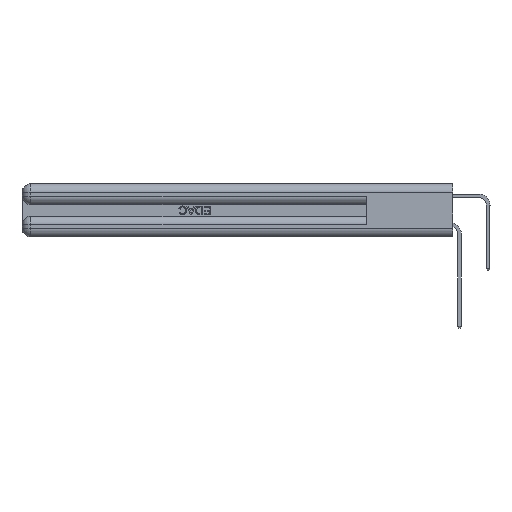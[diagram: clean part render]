
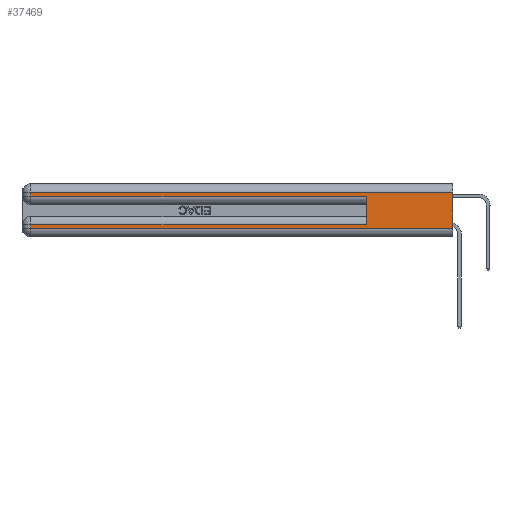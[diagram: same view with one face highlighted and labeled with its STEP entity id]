
A CAD part, left-side view. The second image highlights one B-rep face of the part: STEP entity #37469.
In plain terms, the highlighted planar face has unit normal (-1, 0, 0).
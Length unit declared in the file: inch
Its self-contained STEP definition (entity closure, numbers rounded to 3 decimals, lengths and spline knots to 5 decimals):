
#248 = ORIENTED_EDGE ( 'NONE', *, *, #15402, .T. ) ;
#1178 = ORIENTED_EDGE ( 'NONE', *, *, #9629, .F. ) ;
#1472 = DIRECTION ( 'NONE',  ( 0., 0., -1. ) ) ;
#2189 = EDGE_LOOP ( 'NONE', ( #30689, #19698, #20107, #3870, #1178, #43387, #22085, #248 ) ) ;
#2551 = VERTEX_POINT ( 'NONE', #20019 ) ;
#3870 = ORIENTED_EDGE ( 'NONE', *, *, #19183, .T. ) ;
#5014 = DIRECTION ( 'NONE',  ( 0., -1., 0. ) ) ;
#5498 = VECTOR ( 'NONE', #5014, 39.37008 ) ;
#5734 = CARTESIAN_POINT ( 'NONE',  ( 0., 0., 0.285 ) ) ;
#5761 = CARTESIAN_POINT ( 'NONE',  ( 0., 2.94, 0.31 ) ) ;
#8017 = EDGE_CURVE ( 'NONE', #36345, #47093, #17078, .T. ) ;
#8285 = VECTOR ( 'NONE', #9506, 39.37008 ) ;
#9245 = CARTESIAN_POINT ( 'NONE',  ( 0., 0., 0.37 ) ) ;
#9506 = DIRECTION ( 'NONE',  ( 0., -1., 0. ) ) ;
#9629 = EDGE_CURVE ( 'NONE', #18094, #2551, #47609, .T. ) ;
#10509 = LINE ( 'NONE', #9245, #39495 ) ;
#10948 = VERTEX_POINT ( 'NONE', #39582 ) ;
#11577 = PLANE ( 'NONE',  #39052 ) ;
#11894 = DIRECTION ( 'NONE',  ( 0., 0., -1. ) ) ;
#13617 = EDGE_CURVE ( 'NONE', #10948, #30044, #10509, .T. ) ;
#14584 = DIRECTION ( 'NONE',  ( 0., 0., -1. ) ) ;
#14657 = DIRECTION ( 'NONE',  ( 0., 0., -1. ) ) ;
#15069 = VECTOR ( 'NONE', #44785, 39.37008 ) ;
#15402 = EDGE_CURVE ( 'NONE', #47093, #30044, #16770, .T. ) ;
#16770 = LINE ( 'NONE', #46669, #5498 ) ;
#17068 = CARTESIAN_POINT ( 'NONE',  ( 0., 2.94, 0.085 ) ) ;
#17078 = LINE ( 'NONE', #34968, #21237 ) ;
#17188 = LINE ( 'NONE', #5734, #8285 ) ;
#17857 = CARTESIAN_POINT ( 'NONE',  ( 0., 2.94, 0.06 ) ) ;
#18094 = VERTEX_POINT ( 'NONE', #32365 ) ;
#19183 = EDGE_CURVE ( 'NONE', #25892, #2551, #17188, .T. ) ;
#19698 = ORIENTED_EDGE ( 'NONE', *, *, #41065, .T. ) ;
#20019 = CARTESIAN_POINT ( 'NONE',  ( 0., 0.6, 0.285 ) ) ;
#20107 = ORIENTED_EDGE ( 'NONE', *, *, #40357, .T. ) ;
#21237 = VECTOR ( 'NONE', #14657, 39.37008 ) ;
#21428 = VERTEX_POINT ( 'NONE', #5761 ) ;
#22085 = ORIENTED_EDGE ( 'NONE', *, *, #8017, .T. ) ;
#22688 = CARTESIAN_POINT ( 'NONE',  ( 0., 2.94, 0.285 ) ) ;
#22789 = LINE ( 'NONE', #37031, #15069 ) ;
#23026 = CARTESIAN_POINT ( 'NONE',  ( 0., 0., 0.37 ) ) ;
#23194 = DIRECTION ( 'NONE',  ( 1., 0., 0. ) ) ;
#24087 = DIRECTION ( 'NONE',  ( 0., 1., 0. ) ) ;
#25892 = VERTEX_POINT ( 'NONE', #22688 ) ;
#27527 = LINE ( 'NONE', #45000, #47105 ) ;
#30044 = VERTEX_POINT ( 'NONE', #47420 ) ;
#30689 = ORIENTED_EDGE ( 'NONE', *, *, #13617, .F. ) ;
#32365 = CARTESIAN_POINT ( 'NONE',  ( 0., 0.6, 0.085 ) ) ;
#34968 = CARTESIAN_POINT ( 'NONE',  ( 0., 2.94, 0.37 ) ) ;
#35967 = DIRECTION ( 'NONE',  ( 0., 0., 1. ) ) ;
#36345 = VERTEX_POINT ( 'NONE', #17068 ) ;
#37031 = CARTESIAN_POINT ( 'NONE',  ( 0., 0., 0.31 ) ) ;
#37469 = ADVANCED_FACE ( 'NONE', ( #38488 ), #11577, .F. ) ;
#37547 = VECTOR ( 'NONE', #35967, 39.37008 ) ;
#38294 = EDGE_CURVE ( 'NONE', #18094, #36345, #39005, .T. ) ;
#38488 = FACE_OUTER_BOUND ( 'NONE', #2189, .T. ) ;
#38744 = CARTESIAN_POINT ( 'NONE',  ( 0., 0.6, 0.145 ) ) ;
#39005 = LINE ( 'NONE', #46570, #44969 ) ;
#39052 = AXIS2_PLACEMENT_3D ( 'NONE', #23026, #23194, #11894 ) ;
#39495 = VECTOR ( 'NONE', #1472, 39.37008 ) ;
#39582 = CARTESIAN_POINT ( 'NONE',  ( 0., 0., 0.31 ) ) ;
#40357 = EDGE_CURVE ( 'NONE', #21428, #25892, #27527, .T. ) ;
#41065 = EDGE_CURVE ( 'NONE', #10948, #21428, #22789, .T. ) ;
#43387 = ORIENTED_EDGE ( 'NONE', *, *, #38294, .T. ) ;
#44785 = DIRECTION ( 'NONE',  ( 0., 1., 0. ) ) ;
#44969 = VECTOR ( 'NONE', #24087, 39.37008 ) ;
#45000 = CARTESIAN_POINT ( 'NONE',  ( 0., 2.94, 0.37 ) ) ;
#46570 = CARTESIAN_POINT ( 'NONE',  ( 0., 0., 0.085 ) ) ;
#46669 = CARTESIAN_POINT ( 'NONE',  ( 0., 0., 0.06 ) ) ;
#47093 = VERTEX_POINT ( 'NONE', #17857 ) ;
#47105 = VECTOR ( 'NONE', #14584, 39.37008 ) ;
#47420 = CARTESIAN_POINT ( 'NONE',  ( 0., 0., 0.06 ) ) ;
#47609 = LINE ( 'NONE', #38744, #37547 ) ;
